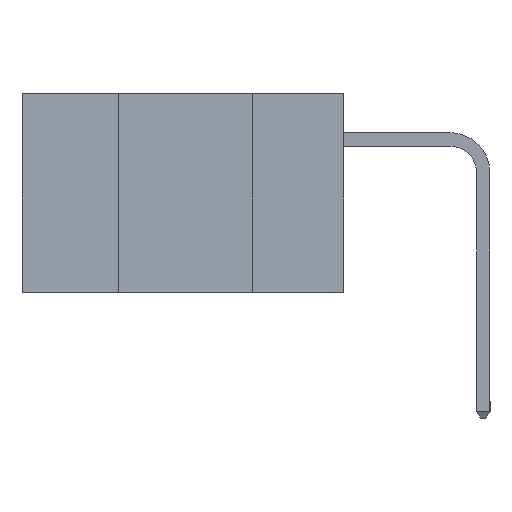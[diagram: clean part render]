
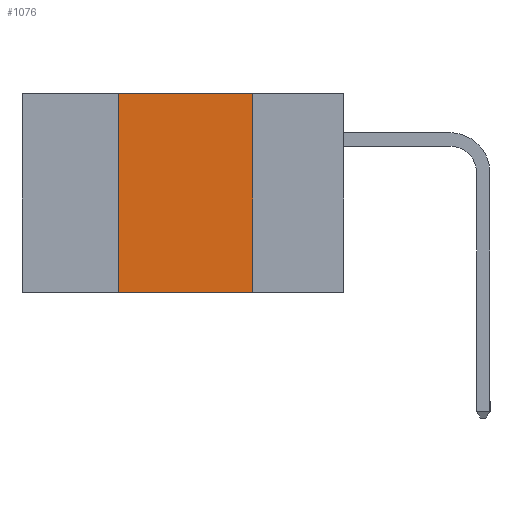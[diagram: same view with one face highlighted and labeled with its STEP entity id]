
A CAD part, left-side view. The second image highlights one B-rep face of the part: STEP entity #1076.
In plain terms, the highlighted planar face has unit normal (-1, 0, 0).
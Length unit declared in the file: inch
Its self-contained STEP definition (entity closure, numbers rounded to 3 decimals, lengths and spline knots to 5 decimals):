
#83 = DIRECTION ( 'NONE',  ( 0., -1., 0. ) ) ;
#475 = LINE ( 'NONE', #2466, #2804 ) ;
#584 = ORIENTED_EDGE ( 'NONE', *, *, #9297, .F. ) ;
#771 = VERTEX_POINT ( 'NONE', #3909 ) ;
#957 = VECTOR ( 'NONE', #83, 39.37008 ) ;
#1076 = ADVANCED_FACE ( 'NONE', ( #6665 ), #11058, .F. ) ;
#2466 = CARTESIAN_POINT ( 'NONE',  ( 0., 0.6, 0. ) ) ;
#2804 = VECTOR ( 'NONE', #4371, 39.37008 ) ;
#3228 = VECTOR ( 'NONE', #10920, 39.37008 ) ;
#3237 = CARTESIAN_POINT ( 'NONE',  ( 0., 0.42, -0.37 ) ) ;
#3523 = ORIENTED_EDGE ( 'NONE', *, *, #9549, .F. ) ;
#3617 = ORIENTED_EDGE ( 'NONE', *, *, #6104, .T. ) ;
#3629 = CARTESIAN_POINT ( 'NONE',  ( 0., 0.6, 0. ) ) ;
#3909 = CARTESIAN_POINT ( 'NONE',  ( 0., 0.42, -0.37 ) ) ;
#4326 = AXIS2_PLACEMENT_3D ( 'NONE', #3629, #5948, #7388 ) ;
#4371 = DIRECTION ( 'NONE',  ( 0., -1., 0. ) ) ;
#4679 = EDGE_LOOP ( 'NONE', ( #584, #5637, #3523, #3617 ) ) ;
#5421 = VERTEX_POINT ( 'NONE', #10863 ) ;
#5517 = CARTESIAN_POINT ( 'NONE',  ( 0., 0.17, 0. ) ) ;
#5637 = ORIENTED_EDGE ( 'NONE', *, *, #7911, .F. ) ;
#5754 = LINE ( 'NONE', #3237, #3228 ) ;
#5766 = VERTEX_POINT ( 'NONE', #5517 ) ;
#5948 = DIRECTION ( 'NONE',  ( 1., 0., 0. ) ) ;
#6081 = LINE ( 'NONE', #8347, #957 ) ;
#6104 = EDGE_CURVE ( 'NONE', #771, #9164, #6081, .T. ) ;
#6665 = FACE_OUTER_BOUND ( 'NONE', #4679, .T. ) ;
#7388 = DIRECTION ( 'NONE',  ( 0., 0., -1. ) ) ;
#7543 = DIRECTION ( 'NONE',  ( 0., 0., -1. ) ) ;
#7571 = VECTOR ( 'NONE', #7543, 39.37008 ) ;
#7911 = EDGE_CURVE ( 'NONE', #5421, #5766, #475, .T. ) ;
#8233 = CARTESIAN_POINT ( 'NONE',  ( 0., 0.17, -0.37 ) ) ;
#8347 = CARTESIAN_POINT ( 'NONE',  ( 0., 0.6, -0.37 ) ) ;
#9164 = VERTEX_POINT ( 'NONE', #8233 ) ;
#9297 = EDGE_CURVE ( 'NONE', #5766, #9164, #9746, .T. ) ;
#9549 = EDGE_CURVE ( 'NONE', #771, #5421, #5754, .T. ) ;
#9746 = LINE ( 'NONE', #9950, #7571 ) ;
#9950 = CARTESIAN_POINT ( 'NONE',  ( 0., 0.17, -0.37 ) ) ;
#10863 = CARTESIAN_POINT ( 'NONE',  ( 0., 0.42, 0. ) ) ;
#10920 = DIRECTION ( 'NONE',  ( 0., 0., 1. ) ) ;
#11058 = PLANE ( 'NONE',  #4326 ) ;
